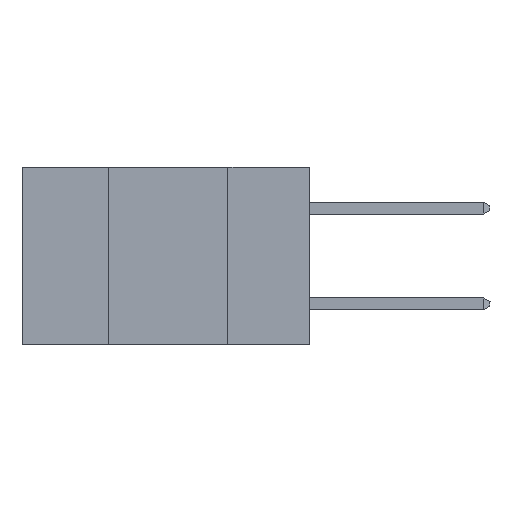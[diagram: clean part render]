
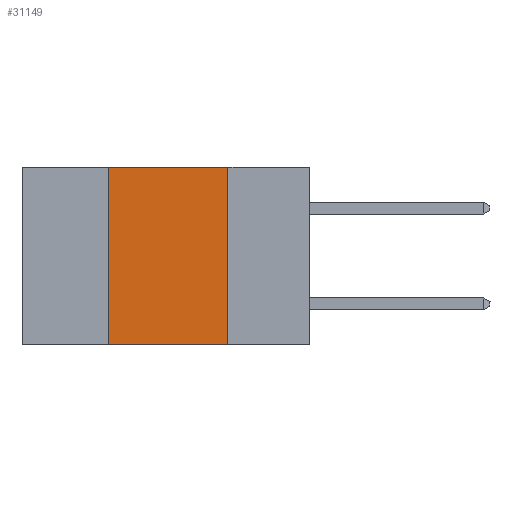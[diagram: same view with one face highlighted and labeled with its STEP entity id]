
A CAD part, left-side view. The second image highlights one B-rep face of the part: STEP entity #31149.
In plain terms, the highlighted planar face has unit normal (-1, 0, 0).
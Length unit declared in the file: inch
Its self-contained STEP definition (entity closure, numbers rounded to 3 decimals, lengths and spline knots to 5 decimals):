
#32 = CARTESIAN_POINT ( 'NONE',  ( 0., 0.17, 0. ) ) ;
#741 = CARTESIAN_POINT ( 'NONE',  ( 0., 0.17, 0. ) ) ;
#1062 = DIRECTION ( 'NONE',  ( 0., -1., 0. ) ) ;
#2044 = CARTESIAN_POINT ( 'NONE',  ( 0., 0.42, -0.37 ) ) ;
#3158 = AXIS2_PLACEMENT_3D ( 'NONE', #33347, #29967, #23411 ) ;
#3629 = CARTESIAN_POINT ( 'NONE',  ( 0., 0.42, 0. ) ) ;
#5071 = VECTOR ( 'NONE', #1062, 39.37008 ) ;
#5464 = VERTEX_POINT ( 'NONE', #26101 ) ;
#8064 = CARTESIAN_POINT ( 'NONE',  ( 0., 0.6, -0.37 ) ) ;
#9271 = EDGE_CURVE ( 'NONE', #5464, #14656, #43785, .T. ) ;
#9886 = VECTOR ( 'NONE', #28258, 39.37008 ) ;
#14656 = VERTEX_POINT ( 'NONE', #32 ) ;
#15264 = VERTEX_POINT ( 'NONE', #30769 ) ;
#15670 = VERTEX_POINT ( 'NONE', #2044 ) ;
#15835 = EDGE_CURVE ( 'NONE', #15670, #15264, #44226, .T. ) ;
#16338 = EDGE_CURVE ( 'NONE', #14656, #15264, #18607, .T. ) ;
#16943 = ORIENTED_EDGE ( 'NONE', *, *, #16338, .F. ) ;
#18607 = LINE ( 'NONE', #741, #27273 ) ;
#21663 = ORIENTED_EDGE ( 'NONE', *, *, #36875, .F. ) ;
#23411 = DIRECTION ( 'NONE',  ( 0., 0., -1. ) ) ;
#25110 = LINE ( 'NONE', #3629, #9886 ) ;
#25400 = DIRECTION ( 'NONE',  ( 0., 0., -1. ) ) ;
#26101 = CARTESIAN_POINT ( 'NONE',  ( 0., 0.42, 0. ) ) ;
#27273 = VECTOR ( 'NONE', #25400, 39.37008 ) ;
#27319 = DIRECTION ( 'NONE',  ( 0., -1., 0. ) ) ;
#28258 = DIRECTION ( 'NONE',  ( 0., 0., 1. ) ) ;
#29967 = DIRECTION ( 'NONE',  ( 1., 0., 0. ) ) ;
#30769 = CARTESIAN_POINT ( 'NONE',  ( 0., 0.17, -0.37 ) ) ;
#31149 = ADVANCED_FACE ( 'NONE', ( #36753 ), #37167, .F. ) ;
#33347 = CARTESIAN_POINT ( 'NONE',  ( 0., 0.6, 0. ) ) ;
#35708 = EDGE_LOOP ( 'NONE', ( #16943, #39740, #21663, #38055 ) ) ;
#36753 = FACE_OUTER_BOUND ( 'NONE', #35708, .T. ) ;
#36875 = EDGE_CURVE ( 'NONE', #15670, #5464, #25110, .T. ) ;
#37167 = PLANE ( 'NONE',  #3158 ) ;
#37236 = CARTESIAN_POINT ( 'NONE',  ( 0., 0.6, 0. ) ) ;
#38055 = ORIENTED_EDGE ( 'NONE', *, *, #15835, .T. ) ;
#39740 = ORIENTED_EDGE ( 'NONE', *, *, #9271, .F. ) ;
#40049 = VECTOR ( 'NONE', #27319, 39.37008 ) ;
#43785 = LINE ( 'NONE', #37236, #40049 ) ;
#44226 = LINE ( 'NONE', #8064, #5071 ) ;
